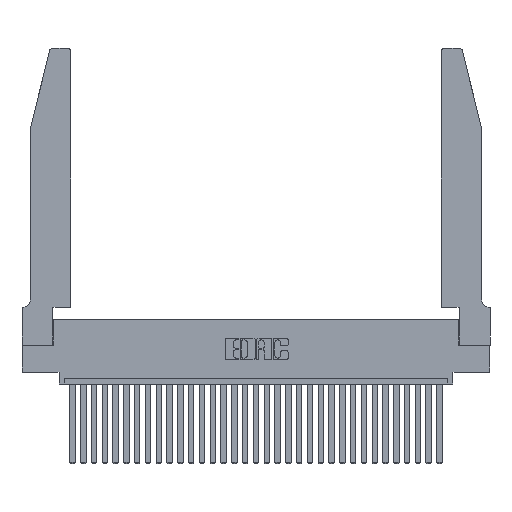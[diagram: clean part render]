
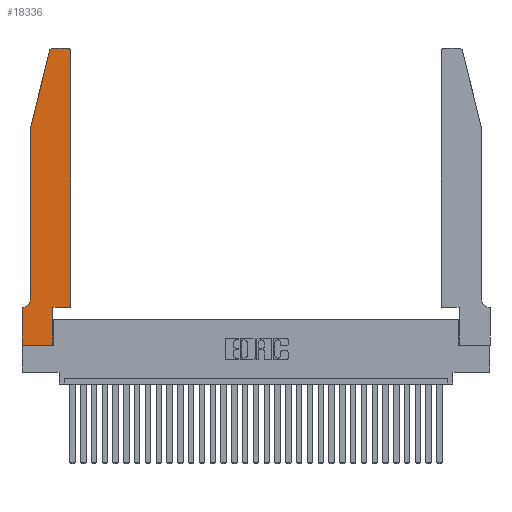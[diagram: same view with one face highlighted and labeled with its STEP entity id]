
A CAD part, top view. The second image highlights one B-rep face of the part: STEP entity #18336.
In plain terms, the highlighted planar face has unit normal (0, 0, 1).
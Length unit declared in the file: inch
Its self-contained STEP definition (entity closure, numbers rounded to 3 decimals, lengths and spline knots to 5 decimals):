
#246 = VECTOR ( 'NONE', #13177, 39.37008 ) ;
#417 = ORIENTED_EDGE ( 'NONE', *, *, #17780, .T. ) ;
#953 = DIRECTION ( 'NONE',  ( 0., 1., 0. ) ) ;
#1345 = CARTESIAN_POINT ( 'NONE',  ( 0.4505, 0.35, 0.37 ) ) ;
#1615 = LINE ( 'NONE', #14206, #8608 ) ;
#2024 = CARTESIAN_POINT ( 'NONE',  ( 0.0055, 0.42, 0.37 ) ) ;
#2310 = CARTESIAN_POINT ( 'NONE',  ( 0.4505, 0.35, 0.37 ) ) ;
#2326 = FACE_OUTER_BOUND ( 'NONE', #5429, .T. ) ;
#2588 = CARTESIAN_POINT ( 'NONE',  ( 0.4505, 0.35, 0.37 ) ) ;
#2994 = LINE ( 'NONE', #12474, #21124 ) ;
#3568 = VERTEX_POINT ( 'NONE', #14439 ) ;
#4232 = DIRECTION ( 'NONE',  ( 1., 0., 0. ) ) ;
#4424 = CARTESIAN_POINT ( 'NONE',  ( 0., 0.35, 0.37 ) ) ;
#4563 = DIRECTION ( 'NONE',  ( 1., 0., 0. ) ) ;
#4822 = CARTESIAN_POINT ( 'NONE',  ( 0.4205, 2.75, 0.37 ) ) ;
#5088 = DIRECTION ( 'NONE',  ( 0., 1., 0. ) ) ;
#5429 = EDGE_LOOP ( 'NONE', ( #31310, #8765, #8520, #31077, #13433, #8617, #19553, #16032, #18965, #19516, #417, #14966 ) ) ;
#6087 = DIRECTION ( 'NONE',  ( -1., 0., 0. ) ) ;
#6450 = AXIS2_PLACEMENT_3D ( 'NONE', #19243, #31769, #4563 ) ;
#6506 = VERTEX_POINT ( 'NONE', #2310 ) ;
#6583 = DIRECTION ( 'NONE',  ( 0., 0., -1. ) ) ;
#6918 = DIRECTION ( 'NONE',  ( 0., 0., 1. ) ) ;
#6920 = LINE ( 'NONE', #16462, #21577 ) ;
#7003 = CARTESIAN_POINT ( 'NONE',  ( 0.2865, 0., 0.37 ) ) ;
#8520 = ORIENTED_EDGE ( 'NONE', *, *, #11635, .T. ) ;
#8572 = VERTEX_POINT ( 'NONE', #19275 ) ;
#8608 = VECTOR ( 'NONE', #4232, 39.37008 ) ;
#8617 = ORIENTED_EDGE ( 'NONE', *, *, #15779, .T. ) ;
#8765 = ORIENTED_EDGE ( 'NONE', *, *, #30533, .T. ) ;
#9990 = VERTEX_POINT ( 'NONE', #14389 ) ;
#10296 = VERTEX_POINT ( 'NONE', #29996 ) ;
#10360 = CARTESIAN_POINT ( 'NONE',  ( 0.4205, 2.72, 0.37 ) ) ;
#10432 = VERTEX_POINT ( 'NONE', #7003 ) ;
#10520 = CARTESIAN_POINT ( 'NONE',  ( 0., 0.35, 0.37 ) ) ;
#10671 = VECTOR ( 'NONE', #20532, 39.37008 ) ;
#11031 = EDGE_CURVE ( 'NONE', #22260, #23089, #23747, .T. ) ;
#11255 = CARTESIAN_POINT ( 'NONE',  ( 0.0755, 2., 0.37 ) ) ;
#11310 = VERTEX_POINT ( 'NONE', #4822 ) ;
#11339 = CARTESIAN_POINT ( 'NONE',  ( 0.2865, 0.35, 0.37 ) ) ;
#11635 = EDGE_CURVE ( 'NONE', #9990, #16614, #28373, .T. ) ;
#11668 = EDGE_CURVE ( 'NONE', #18376, #6506, #31089, .T. ) ;
#12149 = DIRECTION ( 'NONE',  ( -1., 0., 0. ) ) ;
#12474 = CARTESIAN_POINT ( 'NONE',  ( 0.2605, 2.75, 0.37 ) ) ;
#12596 = EDGE_CURVE ( 'NONE', #10296, #19081, #24460, .T. ) ;
#12856 = DIRECTION ( 'NONE',  ( 0., 0., 1. ) ) ;
#12870 = LINE ( 'NONE', #2588, #25167 ) ;
#13177 = DIRECTION ( 'NONE',  ( 0., -1., 0. ) ) ;
#13433 = ORIENTED_EDGE ( 'NONE', *, *, #12596, .T. ) ;
#13830 = AXIS2_PLACEMENT_3D ( 'NONE', #2024, #6583, #29244 ) ;
#14206 = CARTESIAN_POINT ( 'NONE',  ( 0., 0., 0.37 ) ) ;
#14389 = CARTESIAN_POINT ( 'NONE',  ( 0.25487, 2.72718, 0.37 ) ) ;
#14439 = CARTESIAN_POINT ( 'NONE',  ( 0.4505, 2.72, 0.37 ) ) ;
#14719 = CARTESIAN_POINT ( 'NONE',  ( 0.0755, 2., 0.37 ) ) ;
#14966 = ORIENTED_EDGE ( 'NONE', *, *, #28015, .T. ) ;
#15542 = CARTESIAN_POINT ( 'NONE',  ( 0., 0., 0.37 ) ) ;
#15715 = LINE ( 'NONE', #30365, #10671 ) ;
#15779 = EDGE_CURVE ( 'NONE', #19081, #22260, #6920, .T. ) ;
#16032 = ORIENTED_EDGE ( 'NONE', *, *, #31385, .T. ) ;
#16462 = CARTESIAN_POINT ( 'NONE',  ( 0.0755, 0.35, 0.37 ) ) ;
#16614 = VERTEX_POINT ( 'NONE', #11255 ) ;
#16758 = PLANE ( 'NONE',  #25864 ) ;
#17780 = EDGE_CURVE ( 'NONE', #6506, #3568, #12870, .T. ) ;
#18309 = CARTESIAN_POINT ( 'NONE',  ( 0.0055, 0.35, 0.37 ) ) ;
#18336 = ADVANCED_FACE ( 'NONE', ( #2326 ), #16758, .T. ) ;
#18376 = VERTEX_POINT ( 'NONE', #27616 ) ;
#18847 = AXIS2_PLACEMENT_3D ( 'NONE', #10360, #12856, #20258 ) ;
#18924 = CIRCLE ( 'NONE', #18847, 0.03 ) ;
#18965 = ORIENTED_EDGE ( 'NONE', *, *, #27681, .T. ) ;
#19081 = VERTEX_POINT ( 'NONE', #18309 ) ;
#19243 = CARTESIAN_POINT ( 'NONE',  ( 0.284, 2.72, 0.37 ) ) ;
#19275 = CARTESIAN_POINT ( 'NONE',  ( 0.284, 2.75, 0.37 ) ) ;
#19516 = ORIENTED_EDGE ( 'NONE', *, *, #11668, .T. ) ;
#19553 = ORIENTED_EDGE ( 'NONE', *, *, #11031, .T. ) ;
#20258 = DIRECTION ( 'NONE',  ( 1., 0., 0. ) ) ;
#20532 = DIRECTION ( 'NONE',  ( 0., -1., 0. ) ) ;
#20631 = EDGE_CURVE ( 'NONE', #11310, #8572, #2994, .T. ) ;
#21124 = VECTOR ( 'NONE', #12149, 39.37008 ) ;
#21455 = EDGE_CURVE ( 'NONE', #16614, #10296, #15715, .T. ) ;
#21577 = VECTOR ( 'NONE', #6087, 39.37008 ) ;
#22260 = VERTEX_POINT ( 'NONE', #10520 ) ;
#22591 = VECTOR ( 'NONE', #27070, 39.37008 ) ;
#23089 = VERTEX_POINT ( 'NONE', #23742 ) ;
#23742 = CARTESIAN_POINT ( 'NONE',  ( 0., 0., 0.37 ) ) ;
#23747 = LINE ( 'NONE', #15542, #246 ) ;
#23792 = DIRECTION ( 'NONE',  ( 1., 0., 0. ) ) ;
#24072 = CIRCLE ( 'NONE', #6450, 0.03 ) ;
#24166 = DIRECTION ( 'NONE',  ( 1., 0., 0. ) ) ;
#24460 = CIRCLE ( 'NONE', #13830, 0.07 ) ;
#25167 = VECTOR ( 'NONE', #5088, 39.37008 ) ;
#25864 = AXIS2_PLACEMENT_3D ( 'NONE', #4424, #6918, #24166 ) ;
#27070 = DIRECTION ( 'NONE',  ( -0.239, -0.971, 0. ) ) ;
#27616 = CARTESIAN_POINT ( 'NONE',  ( 0.2865, 0.35, 0.37 ) ) ;
#27681 = EDGE_CURVE ( 'NONE', #10432, #18376, #31303, .T. ) ;
#28015 = EDGE_CURVE ( 'NONE', #3568, #11310, #18924, .T. ) ;
#28373 = LINE ( 'NONE', #14719, #22591 ) ;
#28558 = VECTOR ( 'NONE', #953, 39.37008 ) ;
#29244 = DIRECTION ( 'NONE',  ( -1., 0., 0. ) ) ;
#29932 = VECTOR ( 'NONE', #23792, 39.37008 ) ;
#29996 = CARTESIAN_POINT ( 'NONE',  ( 0.0755, 0.42, 0.37 ) ) ;
#30365 = CARTESIAN_POINT ( 'NONE',  ( 0.0755, 2., 0.37 ) ) ;
#30533 = EDGE_CURVE ( 'NONE', #8572, #9990, #24072, .T. ) ;
#31077 = ORIENTED_EDGE ( 'NONE', *, *, #21455, .T. ) ;
#31089 = LINE ( 'NONE', #1345, #29932 ) ;
#31303 = LINE ( 'NONE', #11339, #28558 ) ;
#31310 = ORIENTED_EDGE ( 'NONE', *, *, #20631, .T. ) ;
#31385 = EDGE_CURVE ( 'NONE', #23089, #10432, #1615, .T. ) ;
#31769 = DIRECTION ( 'NONE',  ( 0., 0., 1. ) ) ;
